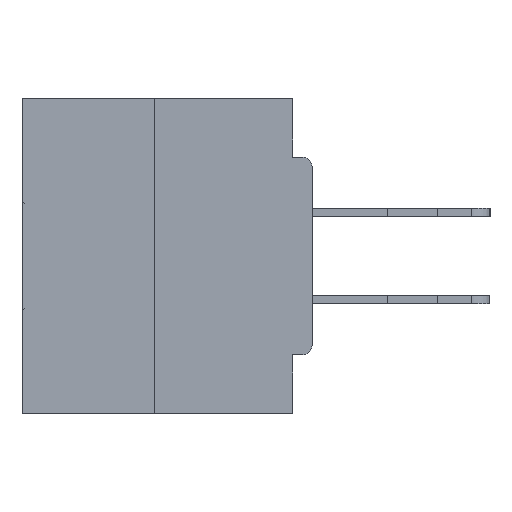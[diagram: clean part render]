
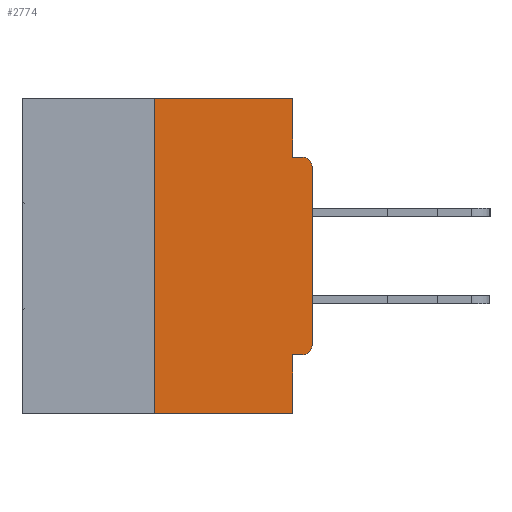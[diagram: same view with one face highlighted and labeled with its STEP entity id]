
A CAD part, left-side view. The second image highlights one B-rep face of the part: STEP entity #2774.
In plain terms, the highlighted planar face has unit normal (-1, 0, 0).
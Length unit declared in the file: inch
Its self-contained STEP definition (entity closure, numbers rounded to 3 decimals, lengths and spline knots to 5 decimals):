
#430 = ORIENTED_EDGE ( 'NONE', *, *, #19957, .F. ) ;
#753 = VERTEX_POINT ( 'NONE', #37839 ) ;
#960 = PLANE ( 'NONE',  #37827 ) ;
#1977 = DIRECTION ( 'NONE',  ( 0., -1., 0. ) ) ;
#2161 = LINE ( 'NONE', #39757, #11145 ) ;
#2774 = ADVANCED_FACE ( 'NONE', ( #22658 ), #960, .F. ) ;
#3117 = EDGE_CURVE ( 'NONE', #41397, #3797, #7550, .T. ) ;
#3699 = VECTOR ( 'NONE', #19572, 39.37008 ) ;
#3797 = VERTEX_POINT ( 'NONE', #14672 ) ;
#4229 = CARTESIAN_POINT ( 'NONE',  ( 0., 0.46, 0. ) ) ;
#4354 = CARTESIAN_POINT ( 'NONE',  ( 0., 0.46, 0. ) ) ;
#4376 = DIRECTION ( 'NONE',  ( 0., 0., -1. ) ) ;
#4565 = EDGE_CURVE ( 'NONE', #25896, #20477, #13406, .T. ) ;
#5424 = LINE ( 'NONE', #8203, #32530 ) ;
#5967 = ORIENTED_EDGE ( 'NONE', *, *, #22908, .F. ) ;
#6367 = VERTEX_POINT ( 'NONE', #14448 ) ;
#7122 = DIRECTION ( 'NONE',  ( 0., 0., -1. ) ) ;
#7550 = LINE ( 'NONE', #24987, #26162 ) ;
#8203 = CARTESIAN_POINT ( 'NONE',  ( 0., 0., 0. ) ) ;
#9220 = CARTESIAN_POINT ( 'NONE',  ( 0., 0.25, -0.5 ) ) ;
#9289 = LINE ( 'NONE', #10205, #20316 ) ;
#9419 = DIRECTION ( 'NONE',  ( 0., 1., 0. ) ) ;
#9447 = CIRCLE ( 'NONE', #9821, 0.015 ) ;
#9774 = CARTESIAN_POINT ( 'NONE',  ( 0., 0., -0.0935 ) ) ;
#9821 = AXIS2_PLACEMENT_3D ( 'NONE', #27292, #27016, #14352 ) ;
#10205 = CARTESIAN_POINT ( 'NONE',  ( 0., 0.031, -0.5 ) ) ;
#10657 = DIRECTION ( 'NONE',  ( 1., 0., 0. ) ) ;
#11145 = VECTOR ( 'NONE', #16613, 39.37008 ) ;
#11152 = CARTESIAN_POINT ( 'NONE',  ( 0., 0.015, -0.4065 ) ) ;
#11527 = CARTESIAN_POINT ( 'NONE',  ( 0., 0.031, -0.0935 ) ) ;
#11660 = DIRECTION ( 'NONE',  ( 0., 0., 1. ) ) ;
#12011 = CARTESIAN_POINT ( 'NONE',  ( 0., 0.25, 0. ) ) ;
#12493 = CARTESIAN_POINT ( 'NONE',  ( 0., 0., -0.4065 ) ) ;
#13406 = LINE ( 'NONE', #12493, #21984 ) ;
#14045 = ORIENTED_EDGE ( 'NONE', *, *, #26358, .T. ) ;
#14352 = DIRECTION ( 'NONE',  ( 0., 0., -1. ) ) ;
#14448 = CARTESIAN_POINT ( 'NONE',  ( 0., 0., -0.3915 ) ) ;
#14672 = CARTESIAN_POINT ( 'NONE',  ( 0., 0.031, -0.5 ) ) ;
#15248 = ORIENTED_EDGE ( 'NONE', *, *, #4565, .F. ) ;
#16613 = DIRECTION ( 'NONE',  ( 0., 0., -1. ) ) ;
#17763 = VERTEX_POINT ( 'NONE', #11527 ) ;
#18260 = LINE ( 'NONE', #9774, #3699 ) ;
#18601 = VECTOR ( 'NONE', #40752, 39.37008 ) ;
#18656 = ORIENTED_EDGE ( 'NONE', *, *, #3117, .T. ) ;
#19572 = DIRECTION ( 'NONE',  ( 0., -1., 0. ) ) ;
#19957 = EDGE_CURVE ( 'NONE', #41397, #41434, #36775, .T. ) ;
#20316 = VECTOR ( 'NONE', #7122, 39.37008 ) ;
#20477 = VERTEX_POINT ( 'NONE', #39960 ) ;
#20852 = DIRECTION ( 'NONE',  ( 0., 0., -1. ) ) ;
#20988 = CARTESIAN_POINT ( 'NONE',  ( 0., 0.015, -0.1085 ) ) ;
#21111 = EDGE_CURVE ( 'NONE', #753, #40733, #27574, .T. ) ;
#21741 = EDGE_CURVE ( 'NONE', #6367, #753, #5424, .T. ) ;
#21804 = ORIENTED_EDGE ( 'NONE', *, *, #24480, .F. ) ;
#21984 = VECTOR ( 'NONE', #9419, 39.37008 ) ;
#22658 = FACE_OUTER_BOUND ( 'NONE', #37098, .T. ) ;
#22908 = EDGE_CURVE ( 'NONE', #20477, #3797, #9289, .T. ) ;
#24480 = EDGE_CURVE ( 'NONE', #38977, #17763, #2161, .T. ) ;
#24987 = CARTESIAN_POINT ( 'NONE',  ( 0., 0.46, -0.5 ) ) ;
#25896 = VERTEX_POINT ( 'NONE', #11152 ) ;
#26081 = ORIENTED_EDGE ( 'NONE', *, *, #21741, .T. ) ;
#26162 = VECTOR ( 'NONE', #1977, 39.37008 ) ;
#26358 = EDGE_CURVE ( 'NONE', #25896, #6367, #9447, .T. ) ;
#26692 = DIRECTION ( 'NONE',  ( 0., 0., 1. ) ) ;
#26833 = ORIENTED_EDGE ( 'NONE', *, *, #37444, .F. ) ;
#27016 = DIRECTION ( 'NONE',  ( -1., 0., 0. ) ) ;
#27292 = CARTESIAN_POINT ( 'NONE',  ( 0., 0.015, -0.3915 ) ) ;
#27574 = CIRCLE ( 'NONE', #41270, 0.015 ) ;
#29177 = ORIENTED_EDGE ( 'NONE', *, *, #41467, .F. ) ;
#30216 = LINE ( 'NONE', #4354, #18601 ) ;
#30592 = DIRECTION ( 'NONE',  ( -1., 0., 0. ) ) ;
#32530 = VECTOR ( 'NONE', #11660, 39.37008 ) ;
#33156 = CARTESIAN_POINT ( 'NONE',  ( 0., 0.25, 0. ) ) ;
#35109 = CARTESIAN_POINT ( 'NONE',  ( 0., 0.031, 0. ) ) ;
#36355 = CARTESIAN_POINT ( 'NONE',  ( 0., 0.015, -0.0935 ) ) ;
#36775 = LINE ( 'NONE', #33156, #37790 ) ;
#37098 = EDGE_LOOP ( 'NONE', ( #26833, #430, #18656, #5967, #15248, #14045, #26081, #38407, #29177, #21804 ) ) ;
#37444 = EDGE_CURVE ( 'NONE', #41434, #38977, #30216, .T. ) ;
#37790 = VECTOR ( 'NONE', #26692, 39.37008 ) ;
#37827 = AXIS2_PLACEMENT_3D ( 'NONE', #4229, #10657, #4376 ) ;
#37839 = CARTESIAN_POINT ( 'NONE',  ( 0., 0., -0.1085 ) ) ;
#38407 = ORIENTED_EDGE ( 'NONE', *, *, #21111, .T. ) ;
#38977 = VERTEX_POINT ( 'NONE', #35109 ) ;
#39757 = CARTESIAN_POINT ( 'NONE',  ( 0., 0.031, 0. ) ) ;
#39960 = CARTESIAN_POINT ( 'NONE',  ( 0., 0.031, -0.4065 ) ) ;
#40733 = VERTEX_POINT ( 'NONE', #36355 ) ;
#40752 = DIRECTION ( 'NONE',  ( 0., -1., 0. ) ) ;
#41270 = AXIS2_PLACEMENT_3D ( 'NONE', #20988, #30592, #20852 ) ;
#41397 = VERTEX_POINT ( 'NONE', #9220 ) ;
#41434 = VERTEX_POINT ( 'NONE', #12011 ) ;
#41467 = EDGE_CURVE ( 'NONE', #17763, #40733, #18260, .T. ) ;
